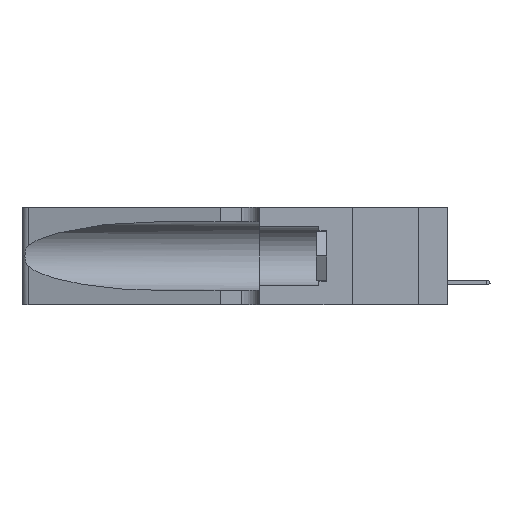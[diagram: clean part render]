
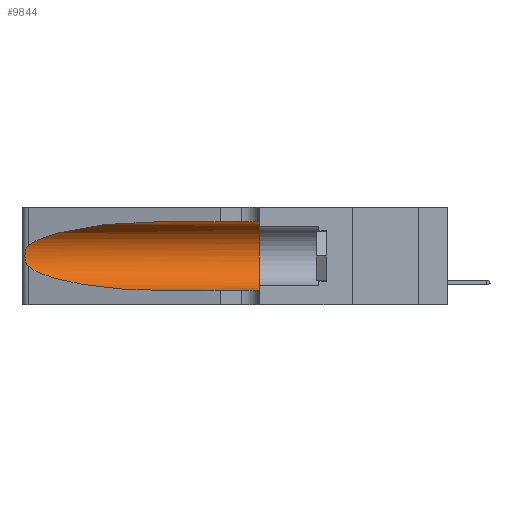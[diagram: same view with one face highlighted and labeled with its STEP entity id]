
A CAD part, left-side view. The second image highlights one B-rep face of the part: STEP entity #9844.
In plain terms, the highlighted cylindrical face has radius 3.308 mm (diameter 6.617 mm), a partial arc.
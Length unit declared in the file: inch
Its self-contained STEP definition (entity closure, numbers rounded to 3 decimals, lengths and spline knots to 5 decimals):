
#1872 = VECTOR ( 'NONE', #34642, 39.37008 ) ;
#2330 = CARTESIAN_POINT ( 'NONE',  ( 0.1305, 0.72297, 0.31525 ) ) ;
#2335 = CARTESIAN_POINT ( 'NONE',  ( 0.25639, 1.23186, 0.15144 ) ) ;
#2986 = ORIENTED_EDGE ( 'NONE', *, *, #25136, .T. ) ;
#3265 = CARTESIAN_POINT ( 'NONE',  ( 0.1305, 0.72297, 0.05475 ) ) ;
#4097 = AXIS2_PLACEMENT_3D ( 'NONE', #18441, #15626, #37002 ) ;
#5470 = VERTEX_POINT ( 'NONE', #20537 ) ;
#6811 = CARTESIAN_POINT ( 'NONE',  ( 0.1305, 1.61858, 0.31525 ) ) ;
#7516 = CARTESIAN_POINT ( 'NONE',  ( 0.25555, 1.22993, 0.14849 ) ) ;
#7889 = VERTEX_POINT ( 'NONE', #15642 ) ;
#8169 = CARTESIAN_POINT ( 'NONE',  ( 0.25555, 1.22994, 0.2215 ) ) ;
#8570 = CARTESIAN_POINT ( 'NONE',  ( 0.25789, 1.23486, 0.15765 ) ) ;
#8641 = ORIENTED_EDGE ( 'NONE', *, *, #24803, .T. ) ;
#9844 = ADVANCED_FACE ( 'NONE', ( #22289 ), #18493, .F. ) ;
#10210 = CARTESIAN_POINT ( 'NONE',  ( 0.1305, 1.61858, 0.05475 ) ) ;
#11129 = CARTESIAN_POINT ( 'NONE',  ( 0.25487, 1.22718, 0.22369 ) ) ;
#11210 = LINE ( 'NONE', #6811, #21216 ) ;
#11256 = CARTESIAN_POINT ( 'NONE',  ( 0.25856, 1.23593, 0.16098 ) ) ;
#11384 = EDGE_CURVE ( 'NONE', #7889, #29585, #14941, .T. ) ;
#11702 = VERTEX_POINT ( 'NONE', #3265 ) ;
#12476 = CARTESIAN_POINT ( 'NONE',  ( 0.1305, 0.35, 0.05475 ) ) ;
#12629 = CARTESIAN_POINT ( 'NONE',  ( 0.1305, 0.35, 0.185 ) ) ;
#13766 = CARTESIAN_POINT ( 'NONE',  ( 0.25487, 1.22718, 0.14631 ) ) ;
#14179 = CARTESIAN_POINT ( 'NONE',  ( 0.25787, 1.23484, 0.2124 ) ) ;
#14941 = B_SPLINE_CURVE_WITH_KNOTS ( 'NONE', 3,
 ( #11129, #8169, #16581, #14179, #32599, #38752, #29524, #20561, #25763, #11256, #8570, #2335, #7516, #29932 ),
 .UNSPECIFIED., .F., .F.,
 ( 4, 2, 2, 2, 2, 2, 4 ),
 ( 0., 0.00027, 0.00053, 0.00107, 0.0016, 0.00187, 0.00214 ),
 .UNSPECIFIED. ) ;
#15002 = EDGE_CURVE ( 'NONE', #5470, #35647, #11210, .T. ) ;
#15088 = CARTESIAN_POINT ( 'NONE',  ( 0.25487, 1.22718, 0.22369 ) ) ;
#15305 = ORIENTED_EDGE ( 'NONE', *, *, #24655, .F. ) ;
#15626 = DIRECTION ( 'NONE',  ( 0., -1., 0. ) ) ;
#15642 = CARTESIAN_POINT ( 'NONE',  ( 0.25487, 1.22718, 0.22369 ) ) ;
#16571 = CARTESIAN_POINT ( 'NONE',  ( 0.2373, 1.15595, 0.08982 ) ) ;
#16581 = CARTESIAN_POINT ( 'NONE',  ( 0.25639, 1.23184, 0.21858 ) ) ;
#16598 = VERTEX_POINT ( 'NONE', #12476 ) ;
#17781 = CARTESIAN_POINT ( 'NONE',  ( 0.18966, 0.96281, 0.31525 ) ) ;
#18097 = CIRCLE ( 'NONE', #37689, 0.13025 ) ;
#18440 = CARTESIAN_POINT ( 'NONE',  ( 0.2373, 1.15595, 0.28018 ) ) ;
#18441 = CARTESIAN_POINT ( 'NONE',  ( 0.1305, 1.61858, 0.185 ) ) ;
#18493 = CYLINDRICAL_SURFACE ( 'NONE', #4097, 0.13025 ) ;
#18760 = DIRECTION ( 'NONE',  ( 0., 0., 1. ) ) ;
#19696 = ORIENTED_EDGE ( 'NONE', *, *, #11384, .T. ) ;
#20537 = CARTESIAN_POINT ( 'NONE',  ( 0.1305, 0.72297, 0.31525 ) ) ;
#20561 = CARTESIAN_POINT ( 'NONE',  ( 0.26075, 1.23896, 0.178 ) ) ;
#21216 = VECTOR ( 'NONE', #25318, 39.37008 ) ;
#22289 = FACE_OUTER_BOUND ( 'NONE', #35415, .T. ) ;
#22346 = LINE ( 'NONE', #10210, #1872 ) ;
#22529 = CARTESIAN_POINT ( 'NONE',  ( 0.1305, 0.35, 0.31525 ) ) ;
#22816 = CARTESIAN_POINT ( 'NONE',  ( 0.18966, 0.96281, 0.05475 ) ) ;
#23650 = ORIENTED_EDGE ( 'NONE', *, *, #27608, .T. ) ;
#24655 = EDGE_CURVE ( 'NONE', #35647, #16598, #18097, .T. ) ;
#24803 = EDGE_CURVE ( 'NONE', #11702, #16598, #22346, .T. ) ;
#25136 = EDGE_CURVE ( 'NONE', #5470, #7889, #31587, .T. ) ;
#25318 = DIRECTION ( 'NONE',  ( 0., -1., 0. ) ) ;
#25763 = CARTESIAN_POINT ( 'NONE',  ( 0.26017, 1.23833, 0.17102 ) ) ;
#27387 = CARTESIAN_POINT ( 'NONE',  ( 0.25487, 1.22718, 0.14631 ) ) ;
#27401 =( BOUNDED_CURVE ( )  B_SPLINE_CURVE ( 3, ( #13766, #16571, #22816, #28969 ),
 .UNSPECIFIED., .F., .T. ) 
 B_SPLINE_CURVE_WITH_KNOTS ( ( 4, 4 ),
 ( 3.44316, 4.71239 ),
 .UNSPECIFIED. ) 
 CURVE ( )  GEOMETRIC_REPRESENTATION_ITEM ( )  RATIONAL_B_SPLINE_CURVE ( ( 1., 0.87, 0.87, 1. ) ) 
 REPRESENTATION_ITEM ( '' )  );
#27608 = EDGE_CURVE ( 'NONE', #29585, #11702, #27401, .T. ) ;
#28969 = CARTESIAN_POINT ( 'NONE',  ( 0.1305, 0.72297, 0.05475 ) ) ;
#29524 = CARTESIAN_POINT ( 'NONE',  ( 0.26075, 1.23896, 0.19203 ) ) ;
#29585 = VERTEX_POINT ( 'NONE', #27387 ) ;
#29932 = CARTESIAN_POINT ( 'NONE',  ( 0.25487, 1.22718, 0.14631 ) ) ;
#31587 =( BOUNDED_CURVE ( )  B_SPLINE_CURVE ( 3, ( #2330, #17781, #18440, #15088 ),
 .UNSPECIFIED., .F., .T. ) 
 B_SPLINE_CURVE_WITH_KNOTS ( ( 4, 4 ),
 ( 1.5708, 2.84003 ),
 .UNSPECIFIED. ) 
 CURVE ( )  GEOMETRIC_REPRESENTATION_ITEM ( )  RATIONAL_B_SPLINE_CURVE ( ( 1., 0.87, 0.87, 1. ) ) 
 REPRESENTATION_ITEM ( '' )  );
#32599 = CARTESIAN_POINT ( 'NONE',  ( 0.25854, 1.2359, 0.20912 ) ) ;
#33992 = DIRECTION ( 'NONE',  ( 0., 1., 0. ) ) ;
#34642 = DIRECTION ( 'NONE',  ( 0., -1., 0. ) ) ;
#35247 = ORIENTED_EDGE ( 'NONE', *, *, #15002, .F. ) ;
#35415 = EDGE_LOOP ( 'NONE', ( #2986, #19696, #23650, #8641, #15305, #35247 ) ) ;
#35647 = VERTEX_POINT ( 'NONE', #22529 ) ;
#37002 = DIRECTION ( 'NONE',  ( 0., 0., -1. ) ) ;
#37689 = AXIS2_PLACEMENT_3D ( 'NONE', #12629, #33992, #18760 ) ;
#38752 = CARTESIAN_POINT ( 'NONE',  ( 0.26018, 1.23835, 0.19895 ) ) ;
